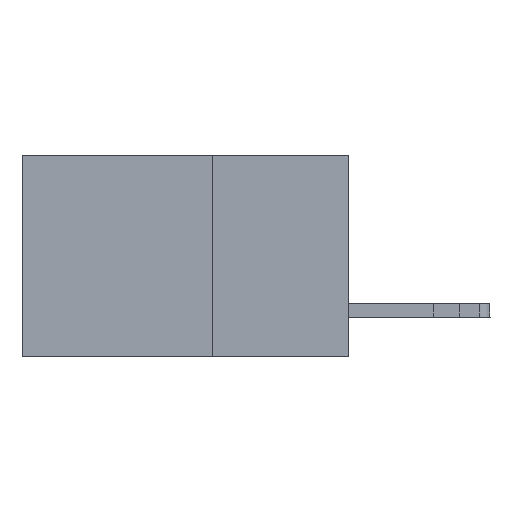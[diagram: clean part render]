
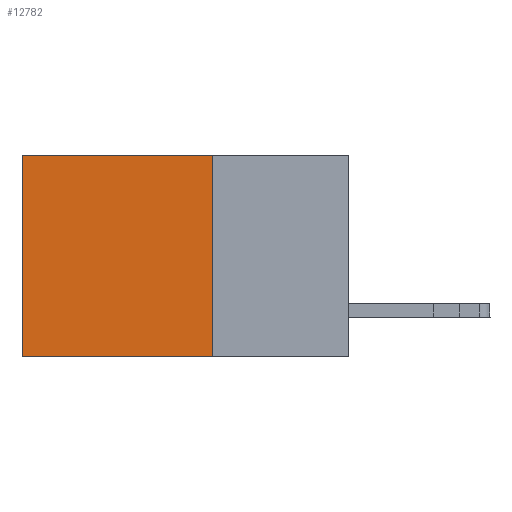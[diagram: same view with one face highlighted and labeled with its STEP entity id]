
A CAD part, left-side view. The second image highlights one B-rep face of the part: STEP entity #12782.
In plain terms, the highlighted planar face has unit normal (-1, 0, 0).
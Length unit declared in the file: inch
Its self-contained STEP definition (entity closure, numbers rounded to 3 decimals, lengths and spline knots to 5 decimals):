
#12 = LINE ( 'NONE', #6057, #4506 ) ;
#455 = EDGE_CURVE ( 'NONE', #21086, #9817, #20215, .T. ) ;
#1267 = VERTEX_POINT ( 'NONE', #22548 ) ;
#1495 = VERTEX_POINT ( 'NONE', #7624 ) ;
#1718 = EDGE_CURVE ( 'NONE', #1495, #1267, #3949, .T. ) ;
#3063 = ORIENTED_EDGE ( 'NONE', *, *, #5767, .T. ) ;
#3949 = LINE ( 'NONE', #9300, #5075 ) ;
#4454 = DIRECTION ( 'NONE',  ( 1., 0., 0. ) ) ;
#4506 = VECTOR ( 'NONE', #9617, 39.37008 ) ;
#4553 = AXIS2_PLACEMENT_3D ( 'NONE', #7938, #4454, #18730 ) ;
#5075 = VECTOR ( 'NONE', #11018, 39.37008 ) ;
#5100 = LINE ( 'NONE', #12343, #17659 ) ;
#5767 = EDGE_CURVE ( 'NONE', #1267, #9817, #5100, .T. ) ;
#6057 = CARTESIAN_POINT ( 'NONE',  ( 0.298, 0.25, 0. ) ) ;
#7624 = CARTESIAN_POINT ( 'NONE',  ( 0.298, 0.25, 0. ) ) ;
#7801 = ORIENTED_EDGE ( 'NONE', *, *, #1718, .T. ) ;
#7938 = CARTESIAN_POINT ( 'NONE',  ( 0.298, 0.25, 0. ) ) ;
#9178 = CARTESIAN_POINT ( 'NONE',  ( 0.298, 0.25, -0.37 ) ) ;
#9300 = CARTESIAN_POINT ( 'NONE',  ( 0.298, 0.25, 0. ) ) ;
#9617 = DIRECTION ( 'NONE',  ( 0., 0., -1. ) ) ;
#9817 = VERTEX_POINT ( 'NONE', #10739 ) ;
#10739 = CARTESIAN_POINT ( 'NONE',  ( 0.298, 0.6, -0.37 ) ) ;
#11018 = DIRECTION ( 'NONE',  ( 0., 1., 0. ) ) ;
#12285 = DIRECTION ( 'NONE',  ( 0., 1., 0. ) ) ;
#12343 = CARTESIAN_POINT ( 'NONE',  ( 0.298, 0.6, 0. ) ) ;
#12439 = PLANE ( 'NONE',  #4553 ) ;
#12664 = DIRECTION ( 'NONE',  ( 0., 0., -1. ) ) ;
#12782 = ADVANCED_FACE ( 'NONE', ( #15477 ), #12439, .F. ) ;
#14934 = ORIENTED_EDGE ( 'NONE', *, *, #19048, .F. ) ;
#15446 = VECTOR ( 'NONE', #12285, 39.37008 ) ;
#15477 = FACE_OUTER_BOUND ( 'NONE', #19544, .T. ) ;
#17659 = VECTOR ( 'NONE', #12664, 39.37008 ) ;
#18730 = DIRECTION ( 'NONE',  ( 0., 0., -1. ) ) ;
#19048 = EDGE_CURVE ( 'NONE', #1495, #21086, #12, .T. ) ;
#19412 = CARTESIAN_POINT ( 'NONE',  ( 0.298, 0.25, -0.37 ) ) ;
#19544 = EDGE_LOOP ( 'NONE', ( #3063, #21154, #14934, #7801 ) ) ;
#20215 = LINE ( 'NONE', #19412, #15446 ) ;
#21086 = VERTEX_POINT ( 'NONE', #9178 ) ;
#21154 = ORIENTED_EDGE ( 'NONE', *, *, #455, .F. ) ;
#22548 = CARTESIAN_POINT ( 'NONE',  ( 0.298, 0.6, 0. ) ) ;
